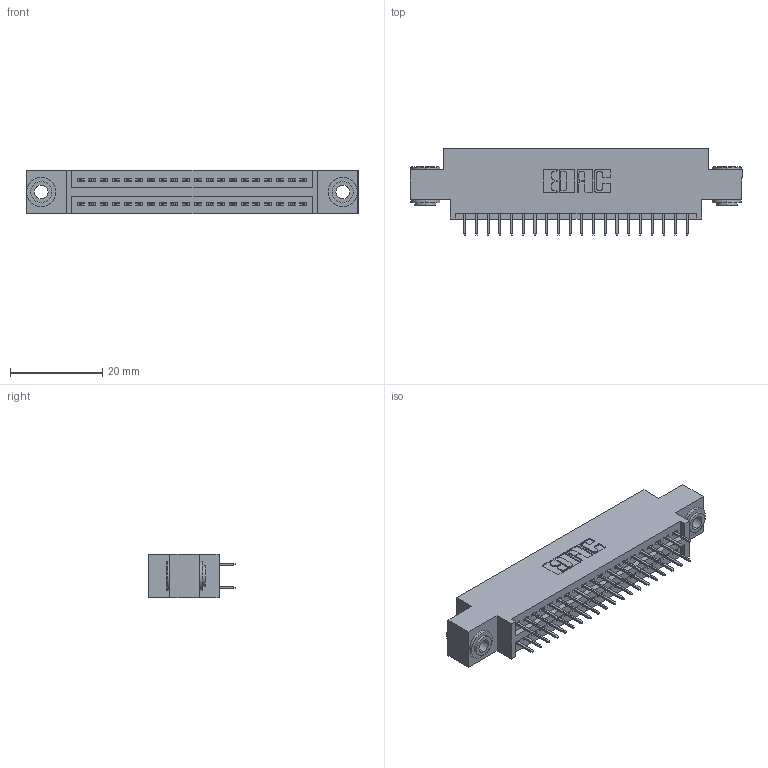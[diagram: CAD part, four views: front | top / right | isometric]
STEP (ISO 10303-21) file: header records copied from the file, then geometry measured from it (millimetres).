
FILE_DESCRIPTION (( 'STEP AP203' ), '1' );
FILE_NAME ('395-040-525-803.STEP', '2020-09-24T02:47:46', ( '' ), ( '' ), 'SwSTEP 2.0', 'SolidWorks 2020', '' );
FILE_SCHEMA (( 'CONFIG_CONTROL_DESIGN' ));
Length unit declared in the file: inch
Products named in the file (4): 345-292-001_345-293-125; 395-040-525-803; 345 Part_0.170 Offset - 0.156 Dia-TH; 345-250-002_345-250-002-102
Assembly tree (43 placements, depth 2):
  395-040-525-803
    345 Part_0.170 Offset - 0.156 Dia-TH
    345-292-001_345-293-125  x40
    345-250-002_345-250-002-102  x2
Bounding box: 72.01 x 18.72 x 9.4 mm (x, y, z)
Volume: 6631 mm3; surface area: 9525.6 mm2
Topology: 43 solids, 43 shells, 2328 faces, 6549 edges, 4202 vertices
Faces by surface type: plane 1654, cylinder 666, cone 8
Entity records: 19510 total; most frequent: CARTESIAN_POINT 3267, ORIENTED_EDGE 3194, DIRECTION 2939, EDGE_CURVE 1597, LINE 1365, VECTOR 1365, VERTEX_POINT 1058, AXIS2_PLACEMENT_3D 787
